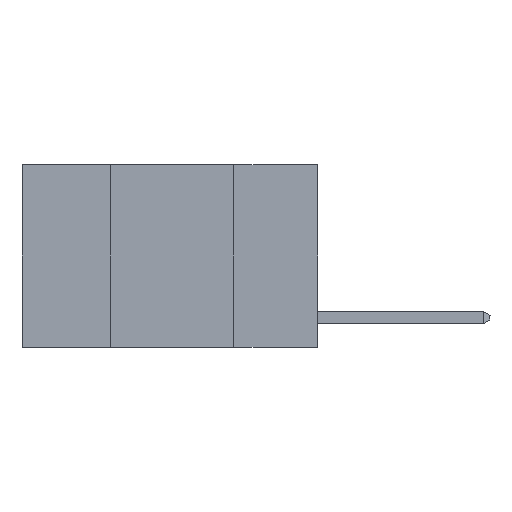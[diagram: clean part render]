
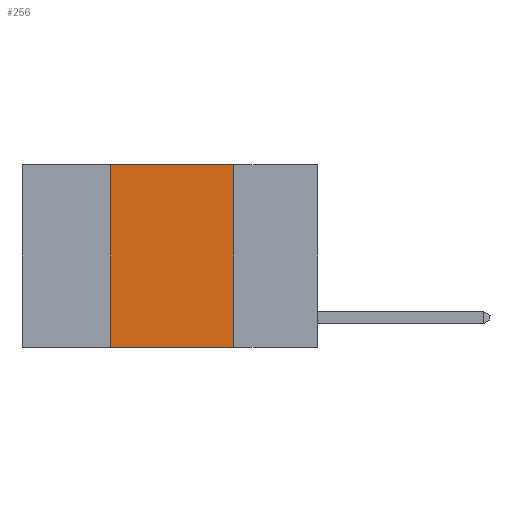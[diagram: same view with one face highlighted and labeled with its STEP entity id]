
A CAD part, left-side view. The second image highlights one B-rep face of the part: STEP entity #256.
In plain terms, the highlighted planar face has unit normal (-1, 0, 0).
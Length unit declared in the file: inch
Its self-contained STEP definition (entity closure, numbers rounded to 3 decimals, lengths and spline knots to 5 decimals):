
#256 = ADVANCED_FACE ( 'NONE', ( #5094 ), #6503, .F. ) ;
#295 = ORIENTED_EDGE ( 'NONE', *, *, #14526, .F. ) ;
#351 = EDGE_CURVE ( 'NONE', #5168, #14813, #10404, .T. ) ;
#1283 = DIRECTION ( 'NONE',  ( 0., 0., -1. ) ) ;
#1385 = EDGE_CURVE ( 'NONE', #5168, #3178, #12037, .T. ) ;
#1875 = VECTOR ( 'NONE', #1283, 39.37008 ) ;
#3093 = VECTOR ( 'NONE', #11068, 39.37008 ) ;
#3178 = VERTEX_POINT ( 'NONE', #14021 ) ;
#3670 = CARTESIAN_POINT ( 'NONE',  ( 0., 0.17, 0. ) ) ;
#4256 = CARTESIAN_POINT ( 'NONE',  ( 0., 0.6, 0. ) ) ;
#4353 = EDGE_LOOP ( 'NONE', ( #6479, #295, #13281, #15139 ) ) ;
#5001 = CARTESIAN_POINT ( 'NONE',  ( 0., 0.42, -0.37 ) ) ;
#5094 = FACE_OUTER_BOUND ( 'NONE', #4353, .T. ) ;
#5168 = VERTEX_POINT ( 'NONE', #5001 ) ;
#5181 = LINE ( 'NONE', #3670, #1875 ) ;
#5507 = CARTESIAN_POINT ( 'NONE',  ( 0., 0.6, -0.37 ) ) ;
#5618 = DIRECTION ( 'NONE',  ( 0., -1., 0. ) ) ;
#6390 = DIRECTION ( 'NONE',  ( 0., 0., -1. ) ) ;
#6391 = DIRECTION ( 'NONE',  ( 1., 0., 0. ) ) ;
#6442 = CARTESIAN_POINT ( 'NONE',  ( 0., 0.6, 0. ) ) ;
#6479 = ORIENTED_EDGE ( 'NONE', *, *, #9944, .F. ) ;
#6503 = PLANE ( 'NONE',  #8027 ) ;
#7569 = VECTOR ( 'NONE', #5618, 39.37008 ) ;
#8027 = AXIS2_PLACEMENT_3D ( 'NONE', #6442, #6391, #6390 ) ;
#8751 = VERTEX_POINT ( 'NONE', #8817 ) ;
#8817 = CARTESIAN_POINT ( 'NONE',  ( 0., 0.17, 0. ) ) ;
#9944 = EDGE_CURVE ( 'NONE', #8751, #14813, #5181, .T. ) ;
#10312 = VECTOR ( 'NONE', #12808, 39.37008 ) ;
#10404 = LINE ( 'NONE', #5507, #7569 ) ;
#10931 = CARTESIAN_POINT ( 'NONE',  ( 0., 0.17, -0.37 ) ) ;
#11068 = DIRECTION ( 'NONE',  ( 0., 0., 1. ) ) ;
#12037 = LINE ( 'NONE', #14596, #3093 ) ;
#12808 = DIRECTION ( 'NONE',  ( 0., -1., 0. ) ) ;
#13281 = ORIENTED_EDGE ( 'NONE', *, *, #1385, .F. ) ;
#13504 = LINE ( 'NONE', #4256, #10312 ) ;
#14021 = CARTESIAN_POINT ( 'NONE',  ( 0., 0.42, 0. ) ) ;
#14526 = EDGE_CURVE ( 'NONE', #3178, #8751, #13504, .T. ) ;
#14596 = CARTESIAN_POINT ( 'NONE',  ( 0., 0.42, 0. ) ) ;
#14813 = VERTEX_POINT ( 'NONE', #10931 ) ;
#15139 = ORIENTED_EDGE ( 'NONE', *, *, #351, .T. ) ;
